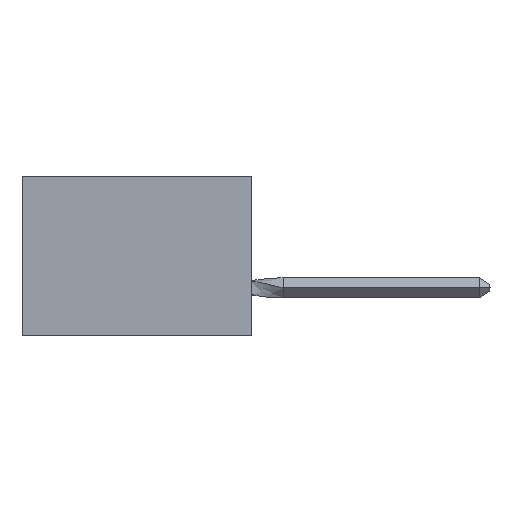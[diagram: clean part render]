
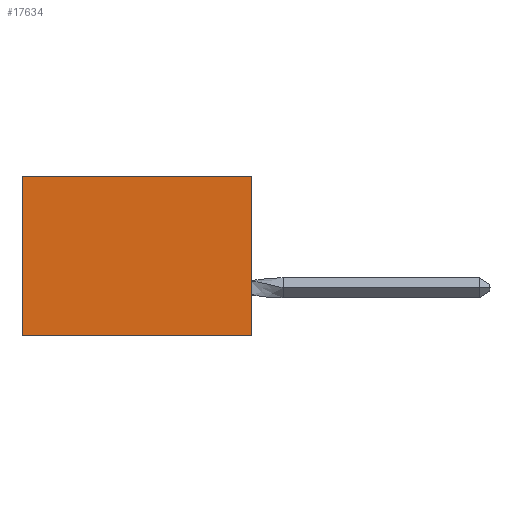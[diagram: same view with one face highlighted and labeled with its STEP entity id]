
A CAD part, left-side view. The second image highlights one B-rep face of the part: STEP entity #17634.
In plain terms, the highlighted planar face has unit normal (-1, 0, 0).
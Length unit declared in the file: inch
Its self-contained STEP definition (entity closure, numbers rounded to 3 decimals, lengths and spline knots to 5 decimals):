
#147 = VERTEX_POINT ( 'NONE', #18535 ) ;
#2064 = ORIENTED_EDGE ( 'NONE', *, *, #14288, .F. ) ;
#2361 = VERTEX_POINT ( 'NONE', #13729 ) ;
#3691 = DIRECTION ( 'NONE',  ( 0., 0., -1. ) ) ;
#4368 = LINE ( 'NONE', #8274, #22103 ) ;
#4427 = VERTEX_POINT ( 'NONE', #21103 ) ;
#4478 = VECTOR ( 'NONE', #17478, 39.37008 ) ;
#4887 = DIRECTION ( 'NONE',  ( 0., 1., 0. ) ) ;
#5588 = LINE ( 'NONE', #7001, #4478 ) ;
#7001 = CARTESIAN_POINT ( 'NONE',  ( 0.305, 0., 0. ) ) ;
#7184 = DIRECTION ( 'NONE',  ( 1., 0., 0. ) ) ;
#7533 = CARTESIAN_POINT ( 'NONE',  ( 0.305, 0., -0.5 ) ) ;
#8274 = CARTESIAN_POINT ( 'NONE',  ( 0.305, 0., -0.5 ) ) ;
#9037 = CARTESIAN_POINT ( 'NONE',  ( 0.305, 0., -0.5 ) ) ;
#10354 = EDGE_CURVE ( 'NONE', #20885, #147, #4368, .T. ) ;
#10716 = VECTOR ( 'NONE', #14609, 39.37008 ) ;
#11890 = AXIS2_PLACEMENT_3D ( 'NONE', #9037, #7184, #3691 ) ;
#12873 = EDGE_CURVE ( 'NONE', #2361, #147, #19824, .T. ) ;
#13054 = VECTOR ( 'NONE', #16647, 39.37008 ) ;
#13729 = CARTESIAN_POINT ( 'NONE',  ( 0.305, 0.72, 0. ) ) ;
#13774 = PLANE ( 'NONE',  #11890 ) ;
#14288 = EDGE_CURVE ( 'NONE', #4427, #20885, #21088, .T. ) ;
#14609 = DIRECTION ( 'NONE',  ( 0., 0., -1. ) ) ;
#14624 = ORIENTED_EDGE ( 'NONE', *, *, #16516, .T. ) ;
#15488 = ORIENTED_EDGE ( 'NONE', *, *, #10354, .F. ) ;
#15872 = EDGE_LOOP ( 'NONE', ( #19980, #15488, #2064, #14624 ) ) ;
#16516 = EDGE_CURVE ( 'NONE', #4427, #2361, #5588, .T. ) ;
#16647 = DIRECTION ( 'NONE',  ( 0., 0., -1. ) ) ;
#17328 = FACE_OUTER_BOUND ( 'NONE', #15872, .T. ) ;
#17478 = DIRECTION ( 'NONE',  ( 0., 1., 0. ) ) ;
#17634 = ADVANCED_FACE ( 'NONE', ( #17328 ), #13774, .F. ) ;
#18535 = CARTESIAN_POINT ( 'NONE',  ( 0.305, 0.72, -0.5 ) ) ;
#19824 = LINE ( 'NONE', #21488, #10716 ) ;
#19980 = ORIENTED_EDGE ( 'NONE', *, *, #12873, .T. ) ;
#20885 = VERTEX_POINT ( 'NONE', #7533 ) ;
#21088 = LINE ( 'NONE', #21893, #13054 ) ;
#21103 = CARTESIAN_POINT ( 'NONE',  ( 0.305, 0., 0. ) ) ;
#21488 = CARTESIAN_POINT ( 'NONE',  ( 0.305, 0.72, -0.5 ) ) ;
#21893 = CARTESIAN_POINT ( 'NONE',  ( 0.305, 0., -0.5 ) ) ;
#22103 = VECTOR ( 'NONE', #4887, 39.37008 ) ;
